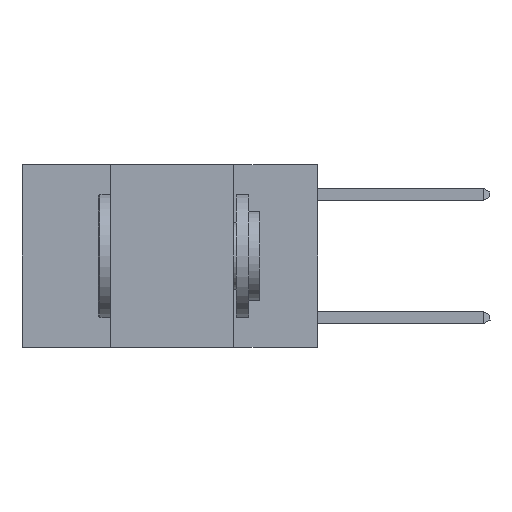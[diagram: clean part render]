
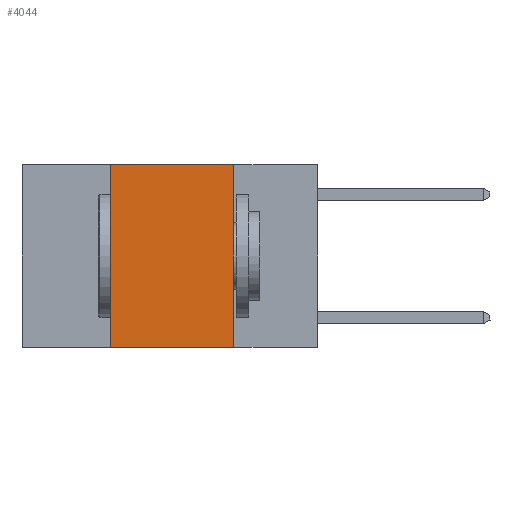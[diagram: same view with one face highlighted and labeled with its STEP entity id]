
A CAD part, left-side view. The second image highlights one B-rep face of the part: STEP entity #4044.
In plain terms, the highlighted planar face has unit normal (-1, 0, 0).
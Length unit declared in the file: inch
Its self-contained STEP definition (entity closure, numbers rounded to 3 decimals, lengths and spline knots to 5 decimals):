
#792 = CARTESIAN_POINT ( 'NONE',  ( 0., 0.42, 0. ) ) ;
#1059 = DIRECTION ( 'NONE',  ( 0., -1., 0. ) ) ;
#1860 = ORIENTED_EDGE ( 'NONE', *, *, #16084, .F. ) ;
#1961 = DIRECTION ( 'NONE',  ( 0., 0., -1. ) ) ;
#2299 = EDGE_CURVE ( 'NONE', #15568, #6945, #15831, .T. ) ;
#3176 = DIRECTION ( 'NONE',  ( 0., -1., 0. ) ) ;
#3676 = VERTEX_POINT ( 'NONE', #16138 ) ;
#4044 = ADVANCED_FACE ( 'NONE', ( #9707 ), #19024, .F. ) ;
#5597 = DIRECTION ( 'NONE',  ( 0., 0., 1. ) ) ;
#5753 = LINE ( 'NONE', #16468, #13013 ) ;
#6833 = EDGE_CURVE ( 'NONE', #17148, #6945, #5753, .T. ) ;
#6945 = VERTEX_POINT ( 'NONE', #10582 ) ;
#7191 = CARTESIAN_POINT ( 'NONE',  ( 0., 0.17, 0. ) ) ;
#7653 = CARTESIAN_POINT ( 'NONE',  ( 0., 0.6, 0. ) ) ;
#7850 = CARTESIAN_POINT ( 'NONE',  ( 0., 0.6, 0. ) ) ;
#7979 = VECTOR ( 'NONE', #5597, 39.37008 ) ;
#9199 = VECTOR ( 'NONE', #3176, 39.37008 ) ;
#9707 = FACE_OUTER_BOUND ( 'NONE', #17491, .T. ) ;
#10582 = CARTESIAN_POINT ( 'NONE',  ( 0., 0.17, -0.37 ) ) ;
#10778 = LINE ( 'NONE', #7653, #9199 ) ;
#11068 = VECTOR ( 'NONE', #1961, 39.37008 ) ;
#12445 = AXIS2_PLACEMENT_3D ( 'NONE', #7850, #14275, #12926 ) ;
#12898 = CARTESIAN_POINT ( 'NONE',  ( 0., 0.42, -0.37 ) ) ;
#12926 = DIRECTION ( 'NONE',  ( 0., 0., -1. ) ) ;
#13013 = VECTOR ( 'NONE', #1059, 39.37008 ) ;
#13331 = LINE ( 'NONE', #792, #7979 ) ;
#14275 = DIRECTION ( 'NONE',  ( 1., 0., 0. ) ) ;
#15568 = VERTEX_POINT ( 'NONE', #7191 ) ;
#15831 = LINE ( 'NONE', #17471, #11068 ) ;
#16084 = EDGE_CURVE ( 'NONE', #3676, #15568, #10778, .T. ) ;
#16138 = CARTESIAN_POINT ( 'NONE',  ( 0., 0.42, 0. ) ) ;
#16468 = CARTESIAN_POINT ( 'NONE',  ( 0., 0.6, -0.37 ) ) ;
#16902 = EDGE_CURVE ( 'NONE', #17148, #3676, #13331, .T. ) ;
#17148 = VERTEX_POINT ( 'NONE', #12898 ) ;
#17471 = CARTESIAN_POINT ( 'NONE',  ( 0., 0.17, 0. ) ) ;
#17491 = EDGE_LOOP ( 'NONE', ( #17858, #1860, #18922, #20322 ) ) ;
#17858 = ORIENTED_EDGE ( 'NONE', *, *, #2299, .F. ) ;
#18922 = ORIENTED_EDGE ( 'NONE', *, *, #16902, .F. ) ;
#19024 = PLANE ( 'NONE',  #12445 ) ;
#20322 = ORIENTED_EDGE ( 'NONE', *, *, #6833, .T. ) ;
